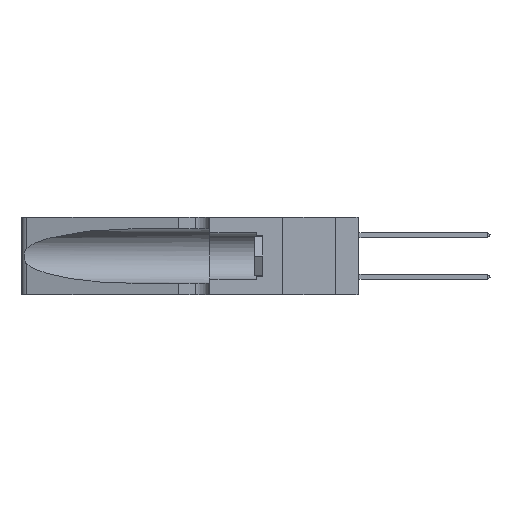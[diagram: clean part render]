
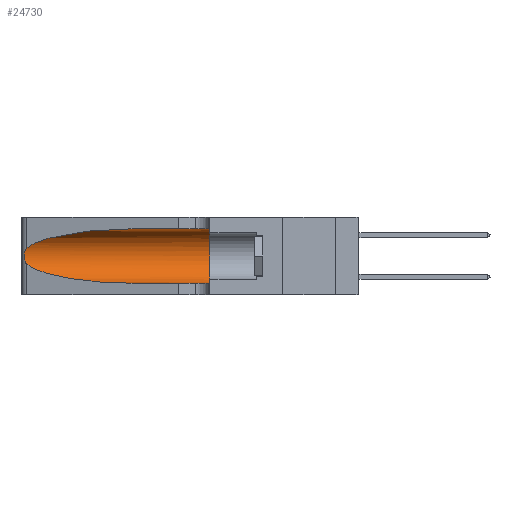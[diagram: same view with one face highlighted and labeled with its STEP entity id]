
A CAD part, left-side view. The second image highlights one B-rep face of the part: STEP entity #24730.
In plain terms, the highlighted cylindrical face has radius 3.308 mm (diameter 6.617 mm), a partial arc.
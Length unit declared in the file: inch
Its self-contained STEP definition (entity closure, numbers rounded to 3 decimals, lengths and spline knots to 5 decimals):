
#421 = CARTESIAN_POINT ( 'NONE',  ( 0.25639, 1.23184, 0.21858 ) ) ;
#811 =( BOUNDED_CURVE ( )  B_SPLINE_CURVE ( 3, ( #32820, #21991, #22585, #6243 ),
 .UNSPECIFIED., .F., .F. ) 
 B_SPLINE_CURVE_WITH_KNOTS ( ( 4, 4 ),
 ( 1.5708, 2.84003 ),
 .UNSPECIFIED. ) 
 CURVE ( )  GEOMETRIC_REPRESENTATION_ITEM ( )  RATIONAL_B_SPLINE_CURVE ( ( 1., 0.87, 0.87, 1. ) ) 
 REPRESENTATION_ITEM ( '' )  );
#2685 = CARTESIAN_POINT ( 'NONE',  ( 0.1305, 0.72297, 0.31525 ) ) ;
#3240 = CARTESIAN_POINT ( 'NONE',  ( 0.25854, 1.2359, 0.20912 ) ) ;
#3420 = VERTEX_POINT ( 'NONE', #10146 ) ;
#3538 = EDGE_LOOP ( 'NONE', ( #11754, #20652, #31851, #22554, #19899, #10150 ) ) ;
#4340 = CARTESIAN_POINT ( 'NONE',  ( 0.1305, 1.61858, 0.185 ) ) ;
#4710 = CARTESIAN_POINT ( 'NONE',  ( 0.25487, 1.22718, 0.14631 ) ) ;
#4957 = EDGE_CURVE ( 'NONE', #3420, #7496, #16266, .T. ) ;
#5674 = EDGE_CURVE ( 'NONE', #33905, #28770, #34744, .T. ) ;
#6011 = CARTESIAN_POINT ( 'NONE',  ( 0.26075, 1.23896, 0.19203 ) ) ;
#6066 = VECTOR ( 'NONE', #10288, 39.37008 ) ;
#6243 = CARTESIAN_POINT ( 'NONE',  ( 0.25487, 1.22718, 0.22369 ) ) ;
#6336 = DIRECTION ( 'NONE',  ( 0., -1., 0. ) ) ;
#7075 = VERTEX_POINT ( 'NONE', #10446 ) ;
#7252 = DIRECTION ( 'NONE',  ( 0., 0., -1. ) ) ;
#7297 =( BOUNDED_CURVE ( )  B_SPLINE_CURVE ( 3, ( #4710, #23799, #26477, #10294 ),
 .UNSPECIFIED., .F., .F. ) 
 B_SPLINE_CURVE_WITH_KNOTS ( ( 4, 4 ),
 ( 3.44316, 4.71239 ),
 .UNSPECIFIED. ) 
 CURVE ( )  GEOMETRIC_REPRESENTATION_ITEM ( )  RATIONAL_B_SPLINE_CURVE ( ( 1., 0.87, 0.87, 1. ) ) 
 REPRESENTATION_ITEM ( '' )  );
#7365 = CARTESIAN_POINT ( 'NONE',  ( 0.1305, 1.61858, 0.31525 ) ) ;
#7496 = VERTEX_POINT ( 'NONE', #22728 ) ;
#8441 = CARTESIAN_POINT ( 'NONE',  ( 0.1305, 0.35, 0.05475 ) ) ;
#8818 = CARTESIAN_POINT ( 'NONE',  ( 0.26017, 1.23833, 0.17102 ) ) ;
#9345 = AXIS2_PLACEMENT_3D ( 'NONE', #4340, #20829, #7252 ) ;
#9476 = FACE_OUTER_BOUND ( 'NONE', #3538, .T. ) ;
#10146 = CARTESIAN_POINT ( 'NONE',  ( 0.25487, 1.22718, 0.22369 ) ) ;
#10150 = ORIENTED_EDGE ( 'NONE', *, *, #22883, .F. ) ;
#10288 = DIRECTION ( 'NONE',  ( 0., -1., 0. ) ) ;
#10294 = CARTESIAN_POINT ( 'NONE',  ( 0.1305, 0.72297, 0.05475 ) ) ;
#10446 = CARTESIAN_POINT ( 'NONE',  ( 0.1305, 0.35, 0.31525 ) ) ;
#10981 = VERTEX_POINT ( 'NONE', #2685 ) ;
#11190 = DIRECTION ( 'NONE',  ( 0., 1., 0. ) ) ;
#11589 = CARTESIAN_POINT ( 'NONE',  ( 0.25789, 1.23486, 0.15765 ) ) ;
#11754 = ORIENTED_EDGE ( 'NONE', *, *, #30769, .T. ) ;
#14207 = CARTESIAN_POINT ( 'NONE',  ( 0.25487, 1.22718, 0.22369 ) ) ;
#14259 = LINE ( 'NONE', #7365, #6066 ) ;
#14322 = CARTESIAN_POINT ( 'NONE',  ( 0.25555, 1.22993, 0.14849 ) ) ;
#16266 = B_SPLINE_CURVE_WITH_KNOTS ( 'NONE', 3,
 ( #14207, #30366, #421, #19625, #3240, #22361, #6011, #25061, #8818, #27777, #11589, #30484, #14322, #33186 ),
 .UNSPECIFIED., .F., .F.,
 ( 4, 2, 2, 2, 2, 2, 4 ),
 ( 0., 0.00027, 0.00053, 0.00107, 0.0016, 0.00187, 0.00214 ),
 .UNSPECIFIED. ) ;
#19625 = CARTESIAN_POINT ( 'NONE',  ( 0.25787, 1.23484, 0.2124 ) ) ;
#19899 = ORIENTED_EDGE ( 'NONE', *, *, #29454, .F. ) ;
#20652 = ORIENTED_EDGE ( 'NONE', *, *, #4957, .T. ) ;
#20829 = DIRECTION ( 'NONE',  ( 0., -1., 0. ) ) ;
#21906 = CIRCLE ( 'NONE', #22881, 0.13025 ) ;
#21991 = CARTESIAN_POINT ( 'NONE',  ( 0.18966, 0.96281, 0.31525 ) ) ;
#22315 = CARTESIAN_POINT ( 'NONE',  ( 0.1305, 0.72297, 0.05475 ) ) ;
#22361 = CARTESIAN_POINT ( 'NONE',  ( 0.26018, 1.23835, 0.19895 ) ) ;
#22554 = ORIENTED_EDGE ( 'NONE', *, *, #5674, .T. ) ;
#22585 = CARTESIAN_POINT ( 'NONE',  ( 0.2373, 1.15595, 0.28018 ) ) ;
#22728 = CARTESIAN_POINT ( 'NONE',  ( 0.25487, 1.22718, 0.14631 ) ) ;
#22881 = AXIS2_PLACEMENT_3D ( 'NONE', #27360, #11190, #30077 ) ;
#22883 = EDGE_CURVE ( 'NONE', #10981, #7075, #14259, .T. ) ;
#23799 = CARTESIAN_POINT ( 'NONE',  ( 0.2373, 1.15595, 0.08982 ) ) ;
#24730 = ADVANCED_FACE ( 'NONE', ( #9476 ), #29378, .F. ) ;
#24785 = EDGE_CURVE ( 'NONE', #7496, #33905, #7297, .T. ) ;
#25061 = CARTESIAN_POINT ( 'NONE',  ( 0.26075, 1.23896, 0.178 ) ) ;
#26477 = CARTESIAN_POINT ( 'NONE',  ( 0.18966, 0.96281, 0.05475 ) ) ;
#27360 = CARTESIAN_POINT ( 'NONE',  ( 0.1305, 0.35, 0.185 ) ) ;
#27575 = VECTOR ( 'NONE', #6336, 39.37008 ) ;
#27777 = CARTESIAN_POINT ( 'NONE',  ( 0.25856, 1.23593, 0.16098 ) ) ;
#28770 = VERTEX_POINT ( 'NONE', #8441 ) ;
#29378 = CYLINDRICAL_SURFACE ( 'NONE', #9345, 0.13025 ) ;
#29454 = EDGE_CURVE ( 'NONE', #7075, #28770, #21906, .T. ) ;
#30077 = DIRECTION ( 'NONE',  ( 0., 0., 1. ) ) ;
#30366 = CARTESIAN_POINT ( 'NONE',  ( 0.25555, 1.22994, 0.2215 ) ) ;
#30484 = CARTESIAN_POINT ( 'NONE',  ( 0.25639, 1.23186, 0.15144 ) ) ;
#30663 = CARTESIAN_POINT ( 'NONE',  ( 0.1305, 1.61858, 0.05475 ) ) ;
#30769 = EDGE_CURVE ( 'NONE', #10981, #3420, #811, .T. ) ;
#31851 = ORIENTED_EDGE ( 'NONE', *, *, #24785, .T. ) ;
#32820 = CARTESIAN_POINT ( 'NONE',  ( 0.1305, 0.72297, 0.31525 ) ) ;
#33186 = CARTESIAN_POINT ( 'NONE',  ( 0.25487, 1.22718, 0.14631 ) ) ;
#33905 = VERTEX_POINT ( 'NONE', #22315 ) ;
#34744 = LINE ( 'NONE', #30663, #27575 ) ;
